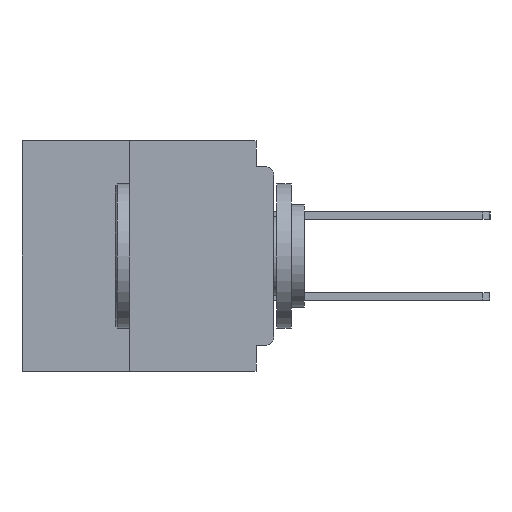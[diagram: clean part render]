
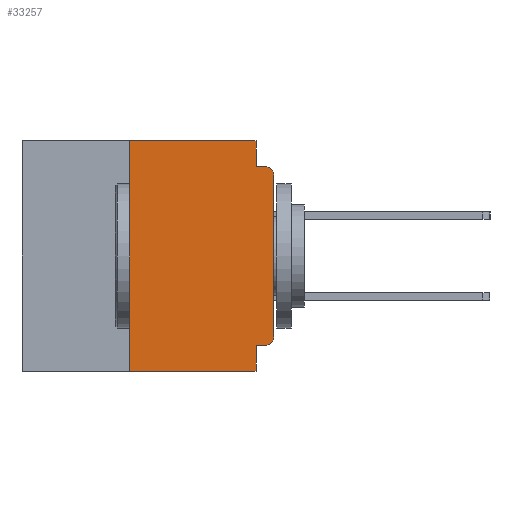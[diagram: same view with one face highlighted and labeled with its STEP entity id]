
A CAD part, left-side view. The second image highlights one B-rep face of the part: STEP entity #33257.
In plain terms, the highlighted planar face has unit normal (-1, 0, 0).
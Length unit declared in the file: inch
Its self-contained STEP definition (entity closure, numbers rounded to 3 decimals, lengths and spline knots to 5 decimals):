
#229 = ORIENTED_EDGE ( 'NONE', *, *, #35373, .F. ) ;
#2703 = CARTESIAN_POINT ( 'NONE',  ( 0., 0.031, -0.4 ) ) ;
#2918 = DIRECTION ( 'NONE',  ( 0., 0., -1. ) ) ;
#3522 = VECTOR ( 'NONE', #63928, 39.37008 ) ;
#3557 = AXIS2_PLACEMENT_3D ( 'NONE', #6316, #41406, #11362 ) ;
#5797 = ORIENTED_EDGE ( 'NONE', *, *, #39285, .F. ) ;
#5952 = VECTOR ( 'NONE', #29262, 39.37008 ) ;
#6316 = CARTESIAN_POINT ( 'NONE',  ( 0., 0.437, 0. ) ) ;
#6826 = ORIENTED_EDGE ( 'NONE', *, *, #52029, .F. ) ;
#7390 = DIRECTION ( 'NONE',  ( -1., 0., 0. ) ) ;
#8188 = EDGE_CURVE ( 'NONE', #12889, #30789, #49459, .T. ) ;
#8635 = ORIENTED_EDGE ( 'NONE', *, *, #22359, .T. ) ;
#8756 = CARTESIAN_POINT ( 'NONE',  ( 0., 0.015, -0.34 ) ) ;
#8835 = CARTESIAN_POINT ( 'NONE',  ( 0., 0.25, -0.4 ) ) ;
#10161 = DIRECTION ( 'NONE',  ( 0., 1., 0. ) ) ;
#10864 = ORIENTED_EDGE ( 'NONE', *, *, #52244, .F. ) ;
#10913 = EDGE_CURVE ( 'NONE', #33612, #24322, #59219, .T. ) ;
#11231 = CARTESIAN_POINT ( 'NONE',  ( 0., 0.031, -0.4 ) ) ;
#11362 = DIRECTION ( 'NONE',  ( 0., 0., -1. ) ) ;
#12889 = VERTEX_POINT ( 'NONE', #35429 ) ;
#13795 = DIRECTION ( 'NONE',  ( 0., 0., -1. ) ) ;
#14315 = LINE ( 'NONE', #15050, #52738 ) ;
#14863 = VECTOR ( 'NONE', #38902, 39.37008 ) ;
#15050 = CARTESIAN_POINT ( 'NONE',  ( 0., 0., -0.045 ) ) ;
#15259 = DIRECTION ( 'NONE',  ( 0., -1., 0. ) ) ;
#15533 = ORIENTED_EDGE ( 'NONE', *, *, #34180, .T. ) ;
#21058 = CARTESIAN_POINT ( 'NONE',  ( 0., 0.25, 0. ) ) ;
#21985 = DIRECTION ( 'NONE',  ( 0., 0., -1. ) ) ;
#22347 = CARTESIAN_POINT ( 'NONE',  ( 0., 0.437, 0. ) ) ;
#22359 = EDGE_CURVE ( 'NONE', #44011, #33612, #62493, .T. ) ;
#24322 = VERTEX_POINT ( 'NONE', #38123 ) ;
#26234 = PLANE ( 'NONE',  #3557 ) ;
#27416 = DIRECTION ( 'NONE',  ( 0., -1., 0. ) ) ;
#28170 = LINE ( 'NONE', #8835, #14863 ) ;
#29262 = DIRECTION ( 'NONE',  ( 0., 0., 1. ) ) ;
#29570 = CARTESIAN_POINT ( 'NONE',  ( 0., 0.015, -0.355 ) ) ;
#30550 = LINE ( 'NONE', #57048, #40045 ) ;
#30789 = VERTEX_POINT ( 'NONE', #11231 ) ;
#31188 = ORIENTED_EDGE ( 'NONE', *, *, #47068, .T. ) ;
#31958 = CIRCLE ( 'NONE', #61457, 0.015 ) ;
#32940 = CARTESIAN_POINT ( 'NONE',  ( 0., 0.031, -0.045 ) ) ;
#33077 = CARTESIAN_POINT ( 'NONE',  ( 0., 0., -0.34 ) ) ;
#33257 = ADVANCED_FACE ( 'NONE', ( #47036 ), #26234, .F. ) ;
#33612 = VERTEX_POINT ( 'NONE', #33077 ) ;
#34007 = CARTESIAN_POINT ( 'NONE',  ( 0., 0.437, -0.4 ) ) ;
#34180 = EDGE_CURVE ( 'NONE', #24322, #38833, #31958, .T. ) ;
#34745 = ORIENTED_EDGE ( 'NONE', *, *, #35092, .F. ) ;
#34809 = VERTEX_POINT ( 'NONE', #32940 ) ;
#35092 = EDGE_CURVE ( 'NONE', #44011, #12889, #43650, .T. ) ;
#35373 = EDGE_CURVE ( 'NONE', #52540, #35864, #64629, .T. ) ;
#35429 = CARTESIAN_POINT ( 'NONE',  ( 0., 0.031, -0.355 ) ) ;
#35864 = VERTEX_POINT ( 'NONE', #46223 ) ;
#37411 = CARTESIAN_POINT ( 'NONE',  ( 0., 0.015, -0.06 ) ) ;
#38121 = VECTOR ( 'NONE', #27416, 39.37008 ) ;
#38123 = CARTESIAN_POINT ( 'NONE',  ( 0., 0., -0.06 ) ) ;
#38833 = VERTEX_POINT ( 'NONE', #51898 ) ;
#38902 = DIRECTION ( 'NONE',  ( 0., 0., 1. ) ) ;
#39285 = EDGE_CURVE ( 'NONE', #34809, #38833, #14315, .T. ) ;
#40045 = VECTOR ( 'NONE', #21985, 39.37008 ) ;
#41091 = VERTEX_POINT ( 'NONE', #60934 ) ;
#41406 = DIRECTION ( 'NONE',  ( 1., 0., 0. ) ) ;
#42082 = VECTOR ( 'NONE', #10161, 39.37008 ) ;
#42145 = ORIENTED_EDGE ( 'NONE', *, *, #8188, .F. ) ;
#42466 = DIRECTION ( 'NONE',  ( 0., 0., -1. ) ) ;
#43650 = LINE ( 'NONE', #55091, #42082 ) ;
#43824 = DIRECTION ( 'NONE',  ( -1., 0., 0. ) ) ;
#44011 = VERTEX_POINT ( 'NONE', #29570 ) ;
#45932 = EDGE_LOOP ( 'NONE', ( #61699, #15533, #5797, #6826, #229, #10864, #31188, #42145, #34745, #8635 ) ) ;
#46223 = CARTESIAN_POINT ( 'NONE',  ( 0., 0.031, 0. ) ) ;
#47036 = FACE_OUTER_BOUND ( 'NONE', #45932, .T. ) ;
#47068 = EDGE_CURVE ( 'NONE', #41091, #30789, #55304, .T. ) ;
#47875 = VECTOR ( 'NONE', #2918, 39.37008 ) ;
#49459 = LINE ( 'NONE', #2703, #47875 ) ;
#51898 = CARTESIAN_POINT ( 'NONE',  ( 0., 0.015, -0.045 ) ) ;
#52029 = EDGE_CURVE ( 'NONE', #35864, #34809, #30550, .T. ) ;
#52244 = EDGE_CURVE ( 'NONE', #41091, #52540, #28170, .T. ) ;
#52540 = VERTEX_POINT ( 'NONE', #21058 ) ;
#52738 = VECTOR ( 'NONE', #15259, 39.37008 ) ;
#54056 = AXIS2_PLACEMENT_3D ( 'NONE', #8756, #43824, #13795 ) ;
#55091 = CARTESIAN_POINT ( 'NONE',  ( 0., 0., -0.355 ) ) ;
#55304 = LINE ( 'NONE', #34007, #3522 ) ;
#57048 = CARTESIAN_POINT ( 'NONE',  ( 0., 0.031, 0. ) ) ;
#59219 = LINE ( 'NONE', #64219, #5952 ) ;
#60934 = CARTESIAN_POINT ( 'NONE',  ( 0., 0.25, -0.4 ) ) ;
#61457 = AXIS2_PLACEMENT_3D ( 'NONE', #37411, #7390, #42466 ) ;
#61699 = ORIENTED_EDGE ( 'NONE', *, *, #10913, .T. ) ;
#62493 = CIRCLE ( 'NONE', #54056, 0.015 ) ;
#63928 = DIRECTION ( 'NONE',  ( 0., -1., 0. ) ) ;
#64219 = CARTESIAN_POINT ( 'NONE',  ( 0., 0., 0. ) ) ;
#64629 = LINE ( 'NONE', #22347, #38121 ) ;
